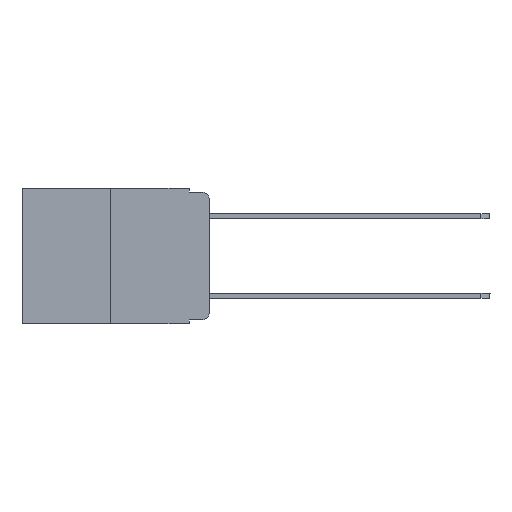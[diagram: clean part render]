
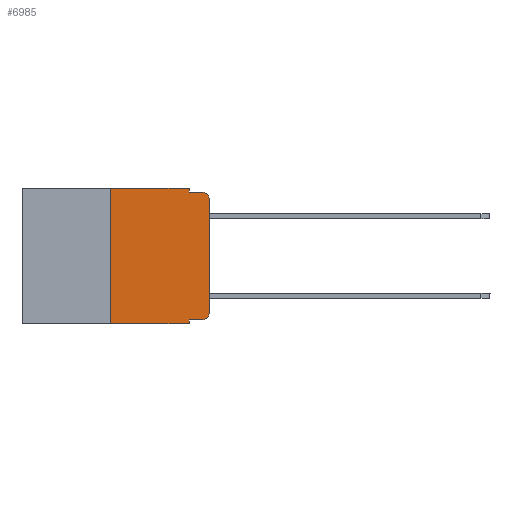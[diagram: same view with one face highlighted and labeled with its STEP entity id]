
A CAD part, left-side view. The second image highlights one B-rep face of the part: STEP entity #6985.
In plain terms, the highlighted planar face has unit normal (-1, 0, 0).
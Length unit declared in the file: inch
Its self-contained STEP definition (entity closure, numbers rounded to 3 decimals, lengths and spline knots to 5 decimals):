
#307 = EDGE_CURVE ( 'NONE', #14240, #6999, #1459, .T. ) ;
#764 = VERTEX_POINT ( 'NONE', #5343 ) ;
#874 = VECTOR ( 'NONE', #4269, 39.37008 ) ;
#1053 = VERTEX_POINT ( 'NONE', #6540 ) ;
#1136 = ORIENTED_EDGE ( 'NONE', *, *, #5284, .F. ) ;
#1182 = DIRECTION ( 'NONE',  ( 0., 0., -1. ) ) ;
#1295 = LINE ( 'NONE', #16915, #9027 ) ;
#1459 = LINE ( 'NONE', #3103, #15620 ) ;
#1594 = CARTESIAN_POINT ( 'NONE',  ( 0., 0.473, 0. ) ) ;
#1634 = CARTESIAN_POINT ( 'NONE',  ( 0., 0., 0. ) ) ;
#2194 = DIRECTION ( 'NONE',  ( 0., 0., -1. ) ) ;
#2594 = ORIENTED_EDGE ( 'NONE', *, *, #13121, .T. ) ;
#2729 = AXIS2_PLACEMENT_3D ( 'NONE', #1594, #13838, #4356 ) ;
#3026 = VERTEX_POINT ( 'NONE', #12565 ) ;
#3092 = CARTESIAN_POINT ( 'NONE',  ( 0., 0.25, 0. ) ) ;
#3103 = CARTESIAN_POINT ( 'NONE',  ( 0., 0.051, -0.01 ) ) ;
#3183 = LINE ( 'NONE', #3092, #17367 ) ;
#3356 = CARTESIAN_POINT ( 'NONE',  ( 0., 0., -0.03 ) ) ;
#3404 = EDGE_LOOP ( 'NONE', ( #16578, #4018, #17279, #1136, #4315, #8784, #7532, #8980, #2594, #11459 ) ) ;
#4018 = ORIENTED_EDGE ( 'NONE', *, *, #8528, .T. ) ;
#4115 = CARTESIAN_POINT ( 'NONE',  ( 0., 0.051, -0.01 ) ) ;
#4269 = DIRECTION ( 'NONE',  ( 0., -1., 0. ) ) ;
#4315 = ORIENTED_EDGE ( 'NONE', *, *, #13788, .F. ) ;
#4331 = EDGE_CURVE ( 'NONE', #13368, #3026, #7994, .T. ) ;
#4356 = DIRECTION ( 'NONE',  ( 0., 0., -1. ) ) ;
#4676 = DIRECTION ( 'NONE',  ( 0., 0., -1. ) ) ;
#4766 = DIRECTION ( 'NONE',  ( 0., -1., 0. ) ) ;
#4822 = VERTEX_POINT ( 'NONE', #6398 ) ;
#4848 = DIRECTION ( 'NONE',  ( -1., 0., 0. ) ) ;
#5284 = EDGE_CURVE ( 'NONE', #764, #14240, #12055, .T. ) ;
#5343 = CARTESIAN_POINT ( 'NONE',  ( 0., 0.051, 0. ) ) ;
#5690 = CARTESIAN_POINT ( 'NONE',  ( 0., 0.25, 0. ) ) ;
#5790 = CARTESIAN_POINT ( 'NONE',  ( 0., 0.473, -0.343 ) ) ;
#5984 = FACE_OUTER_BOUND ( 'NONE', #3404, .T. ) ;
#6398 = CARTESIAN_POINT ( 'NONE',  ( 0., 0.051, -0.343 ) ) ;
#6498 = EDGE_CURVE ( 'NONE', #9372, #4822, #14806, .T. ) ;
#6540 = CARTESIAN_POINT ( 'NONE',  ( 0., 0.25, -0.343 ) ) ;
#6647 = AXIS2_PLACEMENT_3D ( 'NONE', #10529, #4848, #2194 ) ;
#6663 = VERTEX_POINT ( 'NONE', #3356 ) ;
#6905 = LINE ( 'NONE', #9772, #874 ) ;
#6985 = ADVANCED_FACE ( 'NONE', ( #5984 ), #15398, .F. ) ;
#6999 = VERTEX_POINT ( 'NONE', #8380 ) ;
#7532 = ORIENTED_EDGE ( 'NONE', *, *, #12354, .T. ) ;
#7725 = EDGE_CURVE ( 'NONE', #1053, #13698, #3183, .T. ) ;
#7994 = CIRCLE ( 'NONE', #16297, 0.02 ) ;
#8380 = CARTESIAN_POINT ( 'NONE',  ( 0., 0.02, -0.01 ) ) ;
#8491 = DIRECTION ( 'NONE',  ( 0., -1., 0. ) ) ;
#8528 = EDGE_CURVE ( 'NONE', #6663, #6999, #17314, .T. ) ;
#8784 = ORIENTED_EDGE ( 'NONE', *, *, #7725, .F. ) ;
#8876 = DIRECTION ( 'NONE',  ( 0., 0., -1. ) ) ;
#8980 = ORIENTED_EDGE ( 'NONE', *, *, #6498, .F. ) ;
#9027 = VECTOR ( 'NONE', #12569, 39.37008 ) ;
#9372 = VERTEX_POINT ( 'NONE', #10550 ) ;
#9533 = LINE ( 'NONE', #5790, #14035 ) ;
#9772 = CARTESIAN_POINT ( 'NONE',  ( 0., 0.051, -0.333 ) ) ;
#9901 = DIRECTION ( 'NONE',  ( 0., 0., 1. ) ) ;
#10297 = CARTESIAN_POINT ( 'NONE',  ( 0., 0.02, -0.333 ) ) ;
#10529 = CARTESIAN_POINT ( 'NONE',  ( 0., 0.02, -0.03 ) ) ;
#10550 = CARTESIAN_POINT ( 'NONE',  ( 0., 0.051, -0.333 ) ) ;
#11092 = EDGE_CURVE ( 'NONE', #3026, #6663, #17255, .T. ) ;
#11374 = CARTESIAN_POINT ( 'NONE',  ( 0., 0.051, 0. ) ) ;
#11459 = ORIENTED_EDGE ( 'NONE', *, *, #4331, .T. ) ;
#11831 = VECTOR ( 'NONE', #8876, 39.37008 ) ;
#12055 = LINE ( 'NONE', #13015, #11831 ) ;
#12354 = EDGE_CURVE ( 'NONE', #1053, #4822, #9533, .T. ) ;
#12565 = CARTESIAN_POINT ( 'NONE',  ( 0., 0., -0.313 ) ) ;
#12569 = DIRECTION ( 'NONE',  ( 0., -1., 0. ) ) ;
#13015 = CARTESIAN_POINT ( 'NONE',  ( 0., 0.051, 0. ) ) ;
#13121 = EDGE_CURVE ( 'NONE', #9372, #13368, #6905, .T. ) ;
#13141 = VECTOR ( 'NONE', #15384, 39.37008 ) ;
#13368 = VERTEX_POINT ( 'NONE', #10297 ) ;
#13544 = DIRECTION ( 'NONE',  ( -1., 0., 0. ) ) ;
#13698 = VERTEX_POINT ( 'NONE', #5690 ) ;
#13788 = EDGE_CURVE ( 'NONE', #13698, #764, #1295, .T. ) ;
#13838 = DIRECTION ( 'NONE',  ( 1., 0., 0. ) ) ;
#14035 = VECTOR ( 'NONE', #8491, 39.37008 ) ;
#14240 = VERTEX_POINT ( 'NONE', #4115 ) ;
#14593 = VECTOR ( 'NONE', #4676, 39.37008 ) ;
#14806 = LINE ( 'NONE', #11374, #14593 ) ;
#15052 = CARTESIAN_POINT ( 'NONE',  ( 0., 0.02, -0.313 ) ) ;
#15384 = DIRECTION ( 'NONE',  ( 0., 0., 1. ) ) ;
#15398 = PLANE ( 'NONE',  #2729 ) ;
#15620 = VECTOR ( 'NONE', #4766, 39.37008 ) ;
#16297 = AXIS2_PLACEMENT_3D ( 'NONE', #15052, #13544, #1182 ) ;
#16578 = ORIENTED_EDGE ( 'NONE', *, *, #11092, .T. ) ;
#16915 = CARTESIAN_POINT ( 'NONE',  ( 0., 0.473, 0. ) ) ;
#17255 = LINE ( 'NONE', #1634, #13141 ) ;
#17279 = ORIENTED_EDGE ( 'NONE', *, *, #307, .F. ) ;
#17314 = CIRCLE ( 'NONE', #6647, 0.02 ) ;
#17367 = VECTOR ( 'NONE', #9901, 39.37008 ) ;
